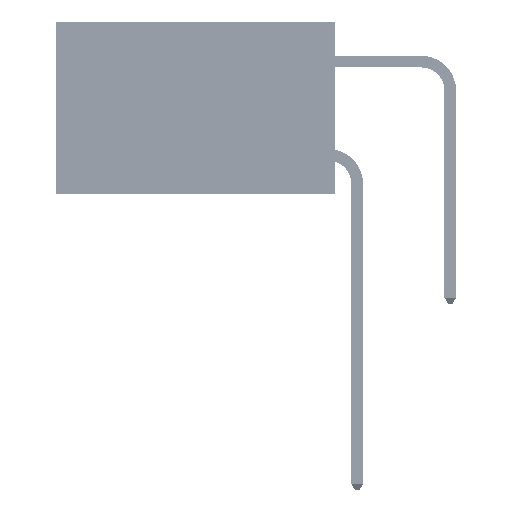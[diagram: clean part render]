
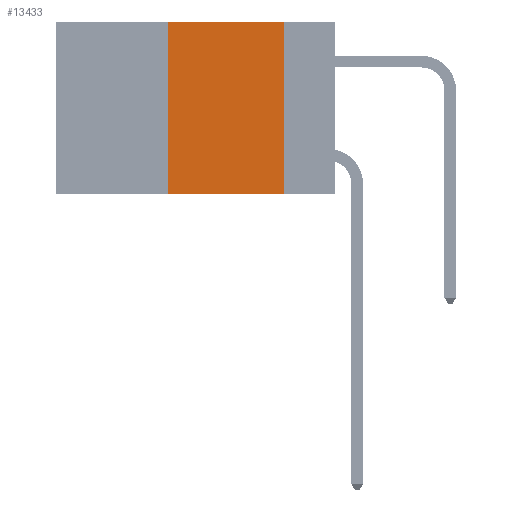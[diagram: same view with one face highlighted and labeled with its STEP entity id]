
A CAD part, left-side view. The second image highlights one B-rep face of the part: STEP entity #13433.
In plain terms, the highlighted planar face has unit normal (-1, 0, 0).
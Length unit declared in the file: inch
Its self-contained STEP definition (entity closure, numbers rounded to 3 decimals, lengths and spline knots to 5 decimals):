
#9 = VECTOR ( 'NONE', #49081, 39.37008 ) ;
#1128 = LINE ( 'NONE', #34088, #29470 ) ;
#4035 = EDGE_LOOP ( 'NONE', ( #6858, #25493, #39146, #29277 ) ) ;
#5538 = CARTESIAN_POINT ( 'NONE',  ( 0., 0.36, 0. ) ) ;
#6858 = ORIENTED_EDGE ( 'NONE', *, *, #24847, .F. ) ;
#7098 = EDGE_CURVE ( 'NONE', #9588, #9799, #24512, .T. ) ;
#7946 = AXIS2_PLACEMENT_3D ( 'NONE', #51477, #14548, #43581 ) ;
#8716 = LINE ( 'NONE', #21355, #9 ) ;
#9588 = VERTEX_POINT ( 'NONE', #39117 ) ;
#9799 = VERTEX_POINT ( 'NONE', #5538 ) ;
#11329 = CARTESIAN_POINT ( 'NONE',  ( 0., 0.11, 0. ) ) ;
#13433 = ADVANCED_FACE ( 'NONE', ( #51209 ), #47021, .F. ) ;
#13489 = CARTESIAN_POINT ( 'NONE',  ( 0., 0.11, -0.37 ) ) ;
#14548 = DIRECTION ( 'NONE',  ( 1., 0., 0. ) ) ;
#15000 = CARTESIAN_POINT ( 'NONE',  ( 0., 0.11, 0. ) ) ;
#16051 = CARTESIAN_POINT ( 'NONE',  ( 0., 0.36, 0. ) ) ;
#17158 = VERTEX_POINT ( 'NONE', #13489 ) ;
#17720 = VECTOR ( 'NONE', #19036, 39.37008 ) ;
#19036 = DIRECTION ( 'NONE',  ( 0., 0., 1. ) ) ;
#19863 = VECTOR ( 'NONE', #26628, 39.37008 ) ;
#20958 = VERTEX_POINT ( 'NONE', #11329 ) ;
#21355 = CARTESIAN_POINT ( 'NONE',  ( 0., 0.6, -0.37 ) ) ;
#24512 = LINE ( 'NONE', #16051, #17720 ) ;
#24847 = EDGE_CURVE ( 'NONE', #20958, #17158, #39304, .T. ) ;
#25493 = ORIENTED_EDGE ( 'NONE', *, *, #40968, .F. ) ;
#26628 = DIRECTION ( 'NONE',  ( 0., 0., -1. ) ) ;
#29277 = ORIENTED_EDGE ( 'NONE', *, *, #41308, .T. ) ;
#29470 = VECTOR ( 'NONE', #30135, 39.37008 ) ;
#30135 = DIRECTION ( 'NONE',  ( 0., -1., 0. ) ) ;
#34088 = CARTESIAN_POINT ( 'NONE',  ( 0., 0.6, 0. ) ) ;
#39117 = CARTESIAN_POINT ( 'NONE',  ( 0., 0.36, -0.37 ) ) ;
#39146 = ORIENTED_EDGE ( 'NONE', *, *, #7098, .F. ) ;
#39304 = LINE ( 'NONE', #15000, #19863 ) ;
#40968 = EDGE_CURVE ( 'NONE', #9799, #20958, #1128, .T. ) ;
#41308 = EDGE_CURVE ( 'NONE', #9588, #17158, #8716, .T. ) ;
#43581 = DIRECTION ( 'NONE',  ( 0., 0., -1. ) ) ;
#47021 = PLANE ( 'NONE',  #7946 ) ;
#49081 = DIRECTION ( 'NONE',  ( 0., -1., 0. ) ) ;
#51209 = FACE_OUTER_BOUND ( 'NONE', #4035, .T. ) ;
#51477 = CARTESIAN_POINT ( 'NONE',  ( 0., 0.6, 0. ) ) ;
